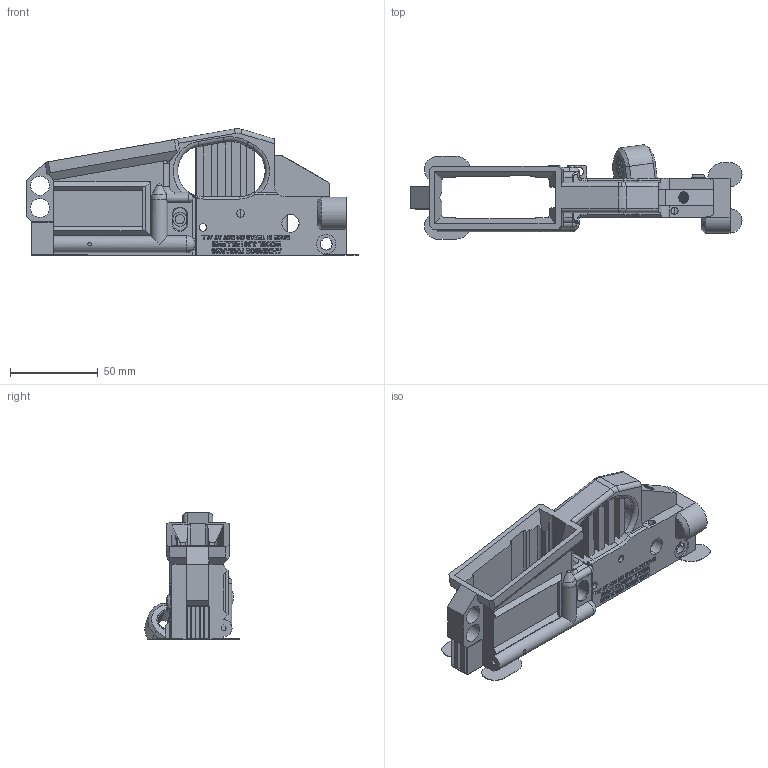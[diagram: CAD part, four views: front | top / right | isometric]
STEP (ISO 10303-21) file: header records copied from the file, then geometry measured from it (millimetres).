
FILE_DESCRIPTION (( 'STEP AP203' ), '1' );
FILE_NAME ('AF-HF-LR-PRT-001-STEP.STEP', '2020-10-04T18:13:46', ( '' ), ( '' ), 'SwSTEP 2.0', 'SolidWorks 2018', '' );
FILE_SCHEMA (( 'CONFIG_CONTROL_DESIGN' ));
Products named in the file (1): AF-HF-LR-PRT-001-STEP
Bounding box: 189.59 x 53.91 x 72.31 mm (x, y, z)
Volume: 100520.1 mm3; surface area: 78211 mm2
Topology: 1 solids, 1 shells, 2754 faces, 7686 edges, 5072 vertices
Faces by surface type: plane 1911, bspline 544, cylinder 256, torus 22, cone 17, sphere 4
Entity records: 165741 total; most frequent: CARTESIAN_POINT 99733, ORIENTED_EDGE 15360, DIRECTION 11035, EDGE_CURVE 7680, LINE 5645, VECTOR 5645, VERTEX_POINT 5071, EDGE_LOOP 2965
